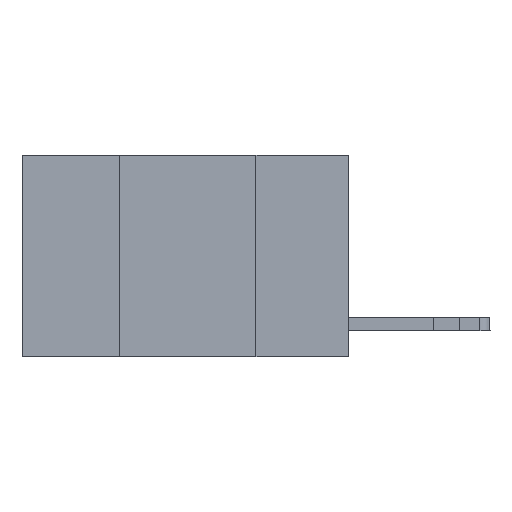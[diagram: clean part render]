
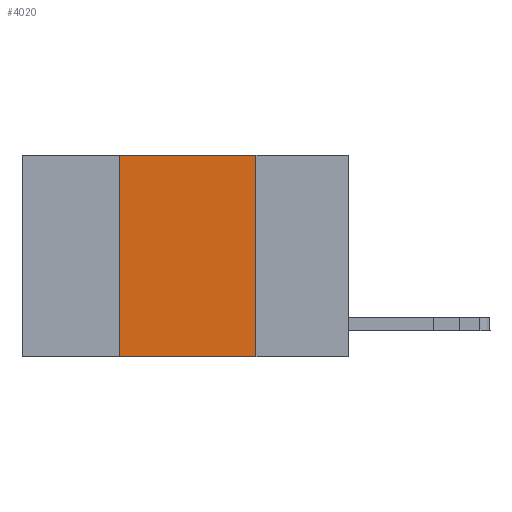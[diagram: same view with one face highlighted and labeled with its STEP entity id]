
A CAD part, left-side view. The second image highlights one B-rep face of the part: STEP entity #4020.
In plain terms, the highlighted planar face has unit normal (-1, 0, 0).
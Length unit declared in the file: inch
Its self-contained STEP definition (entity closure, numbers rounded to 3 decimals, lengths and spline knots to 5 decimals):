
#338 = CARTESIAN_POINT ( 'NONE',  ( 0., 0.42, -0.37 ) ) ;
#1028 = DIRECTION ( 'NONE',  ( 0., 0., -1. ) ) ;
#1091 = PLANE ( 'NONE',  #5908 ) ;
#1227 = EDGE_CURVE ( 'NONE', #8478, #4121, #1497, .T. ) ;
#1497 = LINE ( 'NONE', #9405, #8836 ) ;
#1651 = VECTOR ( 'NONE', #8861, 39.37008 ) ;
#1928 = ORIENTED_EDGE ( 'NONE', *, *, #9100, .F. ) ;
#2453 = CARTESIAN_POINT ( 'NONE',  ( 0., 0.17, -0.37 ) ) ;
#3415 = CARTESIAN_POINT ( 'NONE',  ( 0., 0.17, 0. ) ) ;
#3416 = EDGE_LOOP ( 'NONE', ( #1928, #10433, #12360, #11058 ) ) ;
#3622 = CARTESIAN_POINT ( 'NONE',  ( 0., 0.42, 0. ) ) ;
#4020 = ADVANCED_FACE ( 'NONE', ( #10914 ), #1091, .F. ) ;
#4121 = VERTEX_POINT ( 'NONE', #2453 ) ;
#4151 = CARTESIAN_POINT ( 'NONE',  ( 0., 0.6, 0. ) ) ;
#4618 = VERTEX_POINT ( 'NONE', #11153 ) ;
#5478 = DIRECTION ( 'NONE',  ( 0., 0., -1. ) ) ;
#5604 = VERTEX_POINT ( 'NONE', #3415 ) ;
#5908 = AXIS2_PLACEMENT_3D ( 'NONE', #4151, #10982, #1028 ) ;
#6223 = EDGE_CURVE ( 'NONE', #4618, #5604, #10833, .T. ) ;
#6517 = LINE ( 'NONE', #3622, #11485 ) ;
#7819 = CARTESIAN_POINT ( 'NONE',  ( 0., 0.6, 0. ) ) ;
#8478 = VERTEX_POINT ( 'NONE', #338 ) ;
#8836 = VECTOR ( 'NONE', #10408, 39.37008 ) ;
#8861 = DIRECTION ( 'NONE',  ( 0., -1., 0. ) ) ;
#9100 = EDGE_CURVE ( 'NONE', #5604, #4121, #11302, .T. ) ;
#9367 = VECTOR ( 'NONE', #5478, 39.37008 ) ;
#9405 = CARTESIAN_POINT ( 'NONE',  ( 0., 0.6, -0.37 ) ) ;
#9953 = EDGE_CURVE ( 'NONE', #8478, #4618, #6517, .T. ) ;
#10340 = CARTESIAN_POINT ( 'NONE',  ( 0., 0.17, 0. ) ) ;
#10408 = DIRECTION ( 'NONE',  ( 0., -1., 0. ) ) ;
#10433 = ORIENTED_EDGE ( 'NONE', *, *, #6223, .F. ) ;
#10439 = DIRECTION ( 'NONE',  ( 0., 0., 1. ) ) ;
#10833 = LINE ( 'NONE', #7819, #1651 ) ;
#10914 = FACE_OUTER_BOUND ( 'NONE', #3416, .T. ) ;
#10982 = DIRECTION ( 'NONE',  ( 1., 0., 0. ) ) ;
#11058 = ORIENTED_EDGE ( 'NONE', *, *, #1227, .T. ) ;
#11153 = CARTESIAN_POINT ( 'NONE',  ( 0., 0.42, 0. ) ) ;
#11302 = LINE ( 'NONE', #10340, #9367 ) ;
#11485 = VECTOR ( 'NONE', #10439, 39.37008 ) ;
#12360 = ORIENTED_EDGE ( 'NONE', *, *, #9953, .F. ) ;
